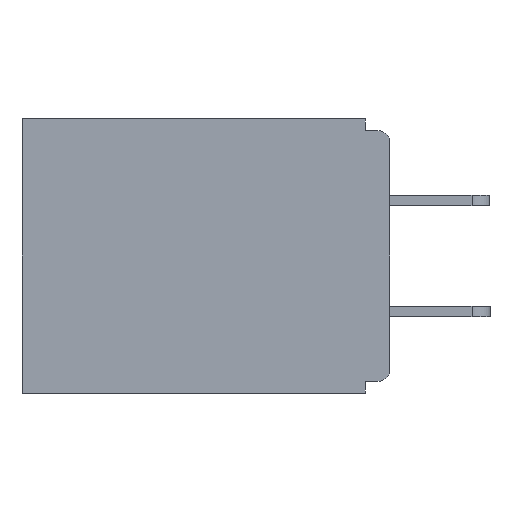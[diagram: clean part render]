
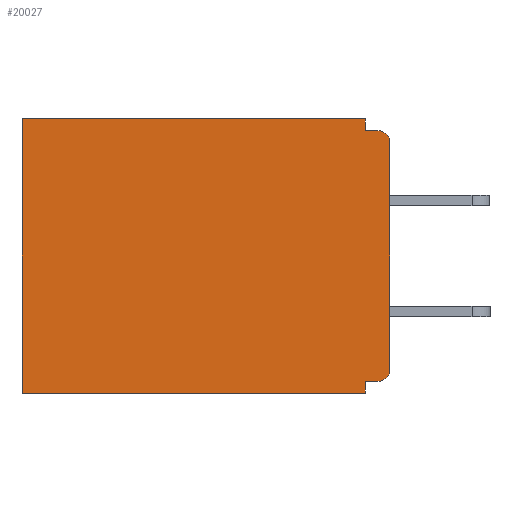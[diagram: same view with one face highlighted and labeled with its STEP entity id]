
A CAD part, left-side view. The second image highlights one B-rep face of the part: STEP entity #20027.
In plain terms, the highlighted planar face has unit normal (-1, 0, 0).
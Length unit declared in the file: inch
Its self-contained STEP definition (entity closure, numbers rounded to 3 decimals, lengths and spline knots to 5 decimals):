
#210 = ORIENTED_EDGE ( 'NONE', *, *, #13971, .F. ) ;
#419 = CARTESIAN_POINT ( 'NONE',  ( 0.298, 0.031, -0.343 ) ) ;
#1116 = VERTEX_POINT ( 'NONE', #11512 ) ;
#1251 = LINE ( 'NONE', #30633, #23784 ) ;
#1352 = DIRECTION ( 'NONE',  ( 1., 0., 0. ) ) ;
#1537 = ORIENTED_EDGE ( 'NONE', *, *, #21710, .F. ) ;
#1559 = CARTESIAN_POINT ( 'NONE',  ( 0.298, 0., -0.03 ) ) ;
#1603 = CARTESIAN_POINT ( 'NONE',  ( 0.298, 0., -0.015 ) ) ;
#1911 = DIRECTION ( 'NONE',  ( 0., -1., 0. ) ) ;
#2063 = CARTESIAN_POINT ( 'NONE',  ( 0.298, 0.46, 0. ) ) ;
#2917 = CARTESIAN_POINT ( 'NONE',  ( 0.298, 0., 0. ) ) ;
#3060 = VERTEX_POINT ( 'NONE', #15132 ) ;
#3548 = CARTESIAN_POINT ( 'NONE',  ( 0.298, 0.015, -0.328 ) ) ;
#3685 = CARTESIAN_POINT ( 'NONE',  ( 0.298, 0., -0.343 ) ) ;
#4551 = CARTESIAN_POINT ( 'NONE',  ( 0.298, 0.031, -0.015 ) ) ;
#4816 = LINE ( 'NONE', #419, #7767 ) ;
#5355 = CIRCLE ( 'NONE', #9895, 0.015 ) ;
#5632 = VECTOR ( 'NONE', #11586, 39.37008 ) ;
#5863 = DIRECTION ( 'NONE',  ( 0., 1., 0. ) ) ;
#6736 = ORIENTED_EDGE ( 'NONE', *, *, #17041, .T. ) ;
#6958 = DIRECTION ( 'NONE',  ( 0., 1., 0. ) ) ;
#7558 = VECTOR ( 'NONE', #1911, 39.37008 ) ;
#7767 = VECTOR ( 'NONE', #28937, 39.37008 ) ;
#8092 = EDGE_CURVE ( 'NONE', #8858, #3060, #17706, .T. ) ;
#8224 = LINE ( 'NONE', #2063, #5632 ) ;
#8240 = CARTESIAN_POINT ( 'NONE',  ( 0.298, 0.031, -0.328 ) ) ;
#8338 = LINE ( 'NONE', #26484, #27598 ) ;
#8685 = EDGE_CURVE ( 'NONE', #15061, #13435, #27621, .T. ) ;
#8858 = VERTEX_POINT ( 'NONE', #13055 ) ;
#9020 = CARTESIAN_POINT ( 'NONE',  ( 0.298, 0.015, -0.313 ) ) ;
#9219 = LINE ( 'NONE', #25035, #11056 ) ;
#9457 = LINE ( 'NONE', #12687, #12055 ) ;
#9739 = DIRECTION ( 'NONE',  ( 0., 1., 0. ) ) ;
#9808 = LINE ( 'NONE', #1603, #7558 ) ;
#9895 = AXIS2_PLACEMENT_3D ( 'NONE', #9020, #11432, #27947 ) ;
#9903 = EDGE_CURVE ( 'NONE', #12690, #1116, #8338, .T. ) ;
#10054 = ORIENTED_EDGE ( 'NONE', *, *, #10057, .F. ) ;
#10057 = EDGE_CURVE ( 'NONE', #12690, #20954, #9457, .T. ) ;
#10503 = CARTESIAN_POINT ( 'NONE',  ( 0.298, 0.015, -0.03 ) ) ;
#10683 = DIRECTION ( 'NONE',  ( 0., 0., -1. ) ) ;
#10989 = FACE_OUTER_BOUND ( 'NONE', #19047, .T. ) ;
#11056 = VECTOR ( 'NONE', #27823, 39.37008 ) ;
#11432 = DIRECTION ( 'NONE',  ( -1., 0., 0. ) ) ;
#11512 = CARTESIAN_POINT ( 'NONE',  ( 0.298, 0.46, 0. ) ) ;
#11586 = DIRECTION ( 'NONE',  ( 0., 0., -1. ) ) ;
#12055 = VECTOR ( 'NONE', #24542, 39.37008 ) ;
#12687 = CARTESIAN_POINT ( 'NONE',  ( 0.298, 0.031, -0.343 ) ) ;
#12690 = VERTEX_POINT ( 'NONE', #27588 ) ;
#12796 = DIRECTION ( 'NONE',  ( -1., 0., 0. ) ) ;
#12840 = VERTEX_POINT ( 'NONE', #8240 ) ;
#13055 = CARTESIAN_POINT ( 'NONE',  ( 0.298, 0.031, -0.343 ) ) ;
#13435 = VERTEX_POINT ( 'NONE', #22293 ) ;
#13971 = EDGE_CURVE ( 'NONE', #12840, #8858, #4816, .T. ) ;
#14561 = VERTEX_POINT ( 'NONE', #27530 ) ;
#15061 = VERTEX_POINT ( 'NONE', #1559 ) ;
#15132 = CARTESIAN_POINT ( 'NONE',  ( 0.298, 0.46, -0.343 ) ) ;
#16329 = ORIENTED_EDGE ( 'NONE', *, *, #9903, .T. ) ;
#16596 = ORIENTED_EDGE ( 'NONE', *, *, #29246, .F. ) ;
#16963 = VECTOR ( 'NONE', #5863, 39.37008 ) ;
#17041 = EDGE_CURVE ( 'NONE', #18634, #14561, #5355, .T. ) ;
#17511 = ORIENTED_EDGE ( 'NONE', *, *, #8685, .T. ) ;
#17706 = LINE ( 'NONE', #3685, #16963 ) ;
#18634 = VERTEX_POINT ( 'NONE', #3548 ) ;
#19047 = EDGE_LOOP ( 'NONE', ( #17511, #1537, #10054, #16329, #24799, #30374, #210, #22255, #6736, #16596 ) ) ;
#19914 = DIRECTION ( 'NONE',  ( 0., 0., -1. ) ) ;
#20027 = ADVANCED_FACE ( 'NONE', ( #10989 ), #28859, .F. ) ;
#20954 = VERTEX_POINT ( 'NONE', #4551 ) ;
#21710 = EDGE_CURVE ( 'NONE', #20954, #13435, #9808, .T. ) ;
#22255 = ORIENTED_EDGE ( 'NONE', *, *, #26667, .F. ) ;
#22293 = CARTESIAN_POINT ( 'NONE',  ( 0.298, 0.015, -0.015 ) ) ;
#23092 = EDGE_CURVE ( 'NONE', #1116, #3060, #8224, .T. ) ;
#23784 = VECTOR ( 'NONE', #6958, 39.37008 ) ;
#24542 = DIRECTION ( 'NONE',  ( 0., 0., -1. ) ) ;
#24799 = ORIENTED_EDGE ( 'NONE', *, *, #23092, .T. ) ;
#25035 = CARTESIAN_POINT ( 'NONE',  ( 0.298, 0., 0. ) ) ;
#25571 = AXIS2_PLACEMENT_3D ( 'NONE', #10503, #12796, #19914 ) ;
#25803 = AXIS2_PLACEMENT_3D ( 'NONE', #2917, #1352, #10683 ) ;
#26484 = CARTESIAN_POINT ( 'NONE',  ( 0.298, 0., 0. ) ) ;
#26667 = EDGE_CURVE ( 'NONE', #18634, #12840, #1251, .T. ) ;
#27530 = CARTESIAN_POINT ( 'NONE',  ( 0.298, 0., -0.313 ) ) ;
#27588 = CARTESIAN_POINT ( 'NONE',  ( 0.298, 0.031, 0. ) ) ;
#27598 = VECTOR ( 'NONE', #9739, 39.37008 ) ;
#27621 = CIRCLE ( 'NONE', #25571, 0.015 ) ;
#27823 = DIRECTION ( 'NONE',  ( 0., 0., -1. ) ) ;
#27947 = DIRECTION ( 'NONE',  ( 0., 0., -1. ) ) ;
#28859 = PLANE ( 'NONE',  #25803 ) ;
#28937 = DIRECTION ( 'NONE',  ( 0., 0., -1. ) ) ;
#29246 = EDGE_CURVE ( 'NONE', #15061, #14561, #9219, .T. ) ;
#30374 = ORIENTED_EDGE ( 'NONE', *, *, #8092, .F. ) ;
#30633 = CARTESIAN_POINT ( 'NONE',  ( 0.298, 0., -0.328 ) ) ;
